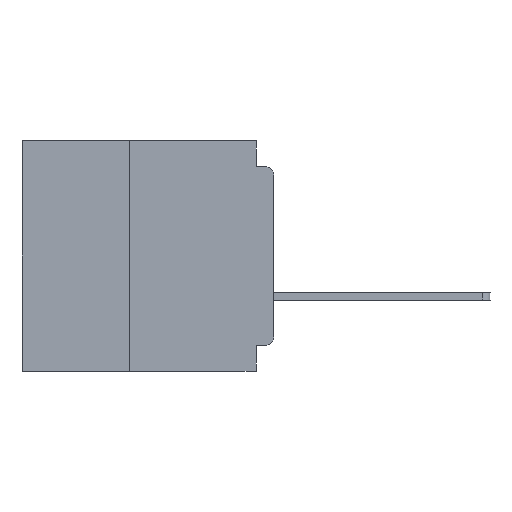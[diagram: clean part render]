
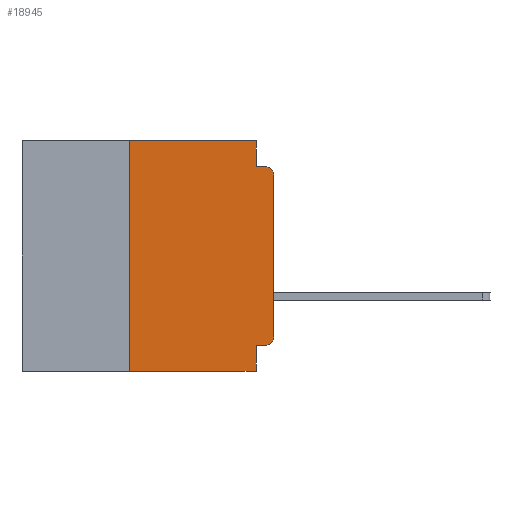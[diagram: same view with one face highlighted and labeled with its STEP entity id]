
A CAD part, left-side view. The second image highlights one B-rep face of the part: STEP entity #18945.
In plain terms, the highlighted planar face has unit normal (-1, 0, 0).
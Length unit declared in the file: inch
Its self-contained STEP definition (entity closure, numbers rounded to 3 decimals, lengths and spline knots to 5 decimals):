
#101 = EDGE_CURVE ( 'NONE', #32713, #12588, #18583, .T. ) ;
#896 = AXIS2_PLACEMENT_3D ( 'NONE', #23411, #59072, #28528 ) ;
#1794 = EDGE_LOOP ( 'NONE', ( #62795, #38743, #32114, #61692, #64506, #14866, #44213, #45406, #34691, #40800 ) ) ;
#2342 = CIRCLE ( 'NONE', #17627, 0.015 ) ;
#4060 = FACE_OUTER_BOUND ( 'NONE', #1794, .T. ) ;
#4484 = DIRECTION ( 'NONE',  ( 0., 0., 1. ) ) ;
#5895 = VERTEX_POINT ( 'NONE', #61476 ) ;
#6324 = CARTESIAN_POINT ( 'NONE',  ( 0., 0.031, -0.355 ) ) ;
#6683 = CARTESIAN_POINT ( 'NONE',  ( 0., 0.031, -0.4 ) ) ;
#7401 = EDGE_CURVE ( 'NONE', #12588, #33260, #17071, .T. ) ;
#8485 = VECTOR ( 'NONE', #48459, 39.37008 ) ;
#9440 = PLANE ( 'NONE',  #18529 ) ;
#10546 = CARTESIAN_POINT ( 'NONE',  ( 0., 0.031, -0.045 ) ) ;
#12139 = EDGE_CURVE ( 'NONE', #5895, #49535, #49329, .T. ) ;
#12588 = VERTEX_POINT ( 'NONE', #6324 ) ;
#12896 = CARTESIAN_POINT ( 'NONE',  ( 0., 0., 0. ) ) ;
#12965 = CARTESIAN_POINT ( 'NONE',  ( 0., 0.437, -0.4 ) ) ;
#13523 = CARTESIAN_POINT ( 'NONE',  ( 0., 0.437, 0. ) ) ;
#13795 = LINE ( 'NONE', #13523, #64766 ) ;
#14866 = ORIENTED_EDGE ( 'NONE', *, *, #18977, .F. ) ;
#17071 = LINE ( 'NONE', #6683, #54611 ) ;
#17177 = CARTESIAN_POINT ( 'NONE',  ( 0., 0.031, -0.4 ) ) ;
#17627 = AXIS2_PLACEMENT_3D ( 'NONE', #55129, #24556, #60209 ) ;
#18002 = DIRECTION ( 'NONE',  ( 0., 0., 1. ) ) ;
#18190 = CARTESIAN_POINT ( 'NONE',  ( 0., 0.25, 0. ) ) ;
#18529 = AXIS2_PLACEMENT_3D ( 'NONE', #45242, #19727, #55442 ) ;
#18583 = LINE ( 'NONE', #37054, #33799 ) ;
#18945 = ADVANCED_FACE ( 'NONE', ( #4060 ), #9440, .F. ) ;
#18977 = EDGE_CURVE ( 'NONE', #29098, #31129, #38517, .T. ) ;
#19727 = DIRECTION ( 'NONE',  ( 1., 0., 0. ) ) ;
#19908 = EDGE_CURVE ( 'NONE', #32713, #20459, #48782, .T. ) ;
#20459 = VERTEX_POINT ( 'NONE', #58356 ) ;
#23145 = VECTOR ( 'NONE', #18002, 39.37008 ) ;
#23411 = CARTESIAN_POINT ( 'NONE',  ( 0., 0.015, -0.34 ) ) ;
#24556 = DIRECTION ( 'NONE',  ( -1., 0., 0. ) ) ;
#24891 = VECTOR ( 'NONE', #4484, 39.37008 ) ;
#28528 = DIRECTION ( 'NONE',  ( 0., 0., -1. ) ) ;
#29039 = CARTESIAN_POINT ( 'NONE',  ( 0., 0., -0.045 ) ) ;
#29098 = VERTEX_POINT ( 'NONE', #64354 ) ;
#29988 = CARTESIAN_POINT ( 'NONE',  ( 0., 0.25, -0.4 ) ) ;
#31129 = VERTEX_POINT ( 'NONE', #18190 ) ;
#32114 = ORIENTED_EDGE ( 'NONE', *, *, #61775, .F. ) ;
#32713 = VERTEX_POINT ( 'NONE', #63775 ) ;
#33260 = VERTEX_POINT ( 'NONE', #17177 ) ;
#33799 = VECTOR ( 'NONE', #36387, 39.37008 ) ;
#33857 = DIRECTION ( 'NONE',  ( 0., -1., 0. ) ) ;
#34691 = ORIENTED_EDGE ( 'NONE', *, *, #101, .F. ) ;
#35777 = EDGE_CURVE ( 'NONE', #55031, #41979, #2342, .T. ) ;
#36387 = DIRECTION ( 'NONE',  ( 0., 1., 0. ) ) ;
#36524 = LINE ( 'NONE', #29039, #63509 ) ;
#37054 = CARTESIAN_POINT ( 'NONE',  ( 0., 0., -0.355 ) ) ;
#38366 = LINE ( 'NONE', #12896, #23145 ) ;
#38517 = LINE ( 'NONE', #29988, #24891 ) ;
#38743 = ORIENTED_EDGE ( 'NONE', *, *, #35777, .T. ) ;
#40800 = ORIENTED_EDGE ( 'NONE', *, *, #19908, .T. ) ;
#41979 = VERTEX_POINT ( 'NONE', #44307 ) ;
#43342 = CARTESIAN_POINT ( 'NONE',  ( 0., 0.031, 0. ) ) ;
#44213 = ORIENTED_EDGE ( 'NONE', *, *, #46408, .T. ) ;
#44307 = CARTESIAN_POINT ( 'NONE',  ( 0., 0.015, -0.045 ) ) ;
#45242 = CARTESIAN_POINT ( 'NONE',  ( 0., 0.437, 0. ) ) ;
#45406 = ORIENTED_EDGE ( 'NONE', *, *, #7401, .F. ) ;
#46408 = EDGE_CURVE ( 'NONE', #29098, #33260, #60974, .T. ) ;
#47638 = DIRECTION ( 'NONE',  ( 0., 0., -1. ) ) ;
#48459 = DIRECTION ( 'NONE',  ( 0., 0., -1. ) ) ;
#48736 = DIRECTION ( 'NONE',  ( 0., -1., 0. ) ) ;
#48782 = CIRCLE ( 'NONE', #896, 0.015 ) ;
#49329 = LINE ( 'NONE', #43342, #8485 ) ;
#49535 = VERTEX_POINT ( 'NONE', #10546 ) ;
#50074 = CARTESIAN_POINT ( 'NONE',  ( 0., 0., -0.06 ) ) ;
#54611 = VECTOR ( 'NONE', #47638, 39.37008 ) ;
#55031 = VERTEX_POINT ( 'NONE', #50074 ) ;
#55129 = CARTESIAN_POINT ( 'NONE',  ( 0., 0.015, -0.06 ) ) ;
#55442 = DIRECTION ( 'NONE',  ( 0., 0., -1. ) ) ;
#55878 = EDGE_CURVE ( 'NONE', #20459, #55031, #38366, .T. ) ;
#58356 = CARTESIAN_POINT ( 'NONE',  ( 0., 0., -0.34 ) ) ;
#59072 = DIRECTION ( 'NONE',  ( -1., 0., 0. ) ) ;
#59607 = EDGE_CURVE ( 'NONE', #31129, #5895, #13795, .T. ) ;
#60209 = DIRECTION ( 'NONE',  ( 0., 0., -1. ) ) ;
#60974 = LINE ( 'NONE', #12965, #62584 ) ;
#61476 = CARTESIAN_POINT ( 'NONE',  ( 0., 0.031, 0. ) ) ;
#61692 = ORIENTED_EDGE ( 'NONE', *, *, #12139, .F. ) ;
#61775 = EDGE_CURVE ( 'NONE', #49535, #41979, #36524, .T. ) ;
#62584 = VECTOR ( 'NONE', #48736, 39.37008 ) ;
#62795 = ORIENTED_EDGE ( 'NONE', *, *, #55878, .T. ) ;
#63509 = VECTOR ( 'NONE', #64633, 39.37008 ) ;
#63775 = CARTESIAN_POINT ( 'NONE',  ( 0., 0.015, -0.355 ) ) ;
#64354 = CARTESIAN_POINT ( 'NONE',  ( 0., 0.25, -0.4 ) ) ;
#64506 = ORIENTED_EDGE ( 'NONE', *, *, #59607, .F. ) ;
#64633 = DIRECTION ( 'NONE',  ( 0., -1., 0. ) ) ;
#64766 = VECTOR ( 'NONE', #33857, 39.37008 ) ;
